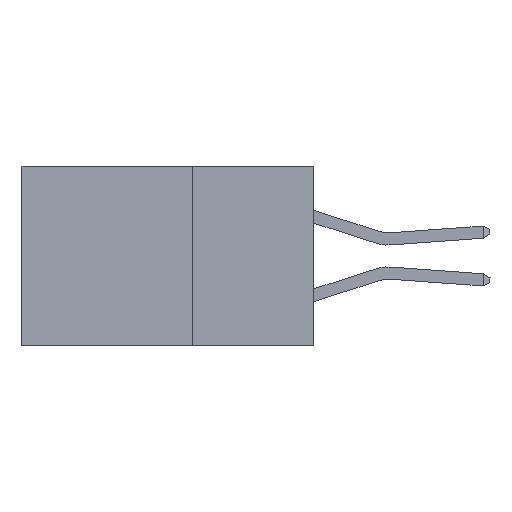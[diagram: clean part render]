
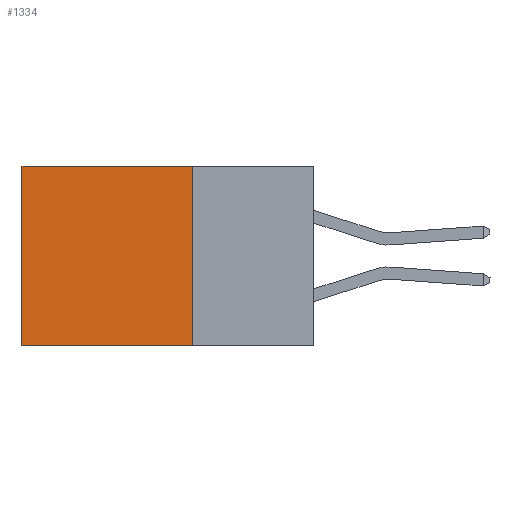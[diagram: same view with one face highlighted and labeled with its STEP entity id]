
A CAD part, left-side view. The second image highlights one B-rep face of the part: STEP entity #1334.
In plain terms, the highlighted planar face has unit normal (-1, 0, 0).
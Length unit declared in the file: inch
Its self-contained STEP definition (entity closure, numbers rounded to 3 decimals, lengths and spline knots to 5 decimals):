
#1334 = ADVANCED_FACE ( 'NONE', ( #14025 ), #2340, .F. ) ;
#2030 = DIRECTION ( 'NONE',  ( 0., 0., -1. ) ) ;
#2246 = DIRECTION ( 'NONE',  ( 1., 0., 0. ) ) ;
#2252 = CARTESIAN_POINT ( 'NONE',  ( 0.2875, 0.25, 0. ) ) ;
#2340 = PLANE ( 'NONE',  #8153 ) ;
#3141 = EDGE_CURVE ( 'NONE', #4321, #3555, #17399, .T. ) ;
#3555 = VERTEX_POINT ( 'NONE', #17788 ) ;
#3614 = CARTESIAN_POINT ( 'NONE',  ( 0.2875, 0.6, 0. ) ) ;
#4321 = VERTEX_POINT ( 'NONE', #3614 ) ;
#4452 = CARTESIAN_POINT ( 'NONE',  ( 0.2875, 0.6, 0. ) ) ;
#6904 = CARTESIAN_POINT ( 'NONE',  ( 0.2875, 0.25, 0. ) ) ;
#7020 = CARTESIAN_POINT ( 'NONE',  ( 0.2875, 0.25, -0.37 ) ) ;
#8153 = AXIS2_PLACEMENT_3D ( 'NONE', #2252, #2246, #2030 ) ;
#8231 = CARTESIAN_POINT ( 'NONE',  ( 0.2875, 0.25, 0. ) ) ;
#9125 = ORIENTED_EDGE ( 'NONE', *, *, #3141, .T. ) ;
#10062 = CARTESIAN_POINT ( 'NONE',  ( 0.2875, 0.25, -0.37 ) ) ;
#10275 = EDGE_CURVE ( 'NONE', #19198, #4321, #13256, .T. ) ;
#10384 = ORIENTED_EDGE ( 'NONE', *, *, #10275, .T. ) ;
#10783 = CARTESIAN_POINT ( 'NONE',  ( 0.2875, 0.25, 0. ) ) ;
#11947 = ORIENTED_EDGE ( 'NONE', *, *, #22106, .F. ) ;
#12358 = VECTOR ( 'NONE', #19217, 39.37008 ) ;
#13256 = LINE ( 'NONE', #6904, #22169 ) ;
#13723 = DIRECTION ( 'NONE',  ( 0., 1., 0. ) ) ;
#14025 = FACE_OUTER_BOUND ( 'NONE', #19454, .T. ) ;
#14488 = VECTOR ( 'NONE', #16910, 39.37008 ) ;
#14865 = ORIENTED_EDGE ( 'NONE', *, *, #15381, .F. ) ;
#15381 = EDGE_CURVE ( 'NONE', #19198, #22263, #19462, .T. ) ;
#15703 = LINE ( 'NONE', #10062, #20112 ) ;
#16910 = DIRECTION ( 'NONE',  ( 0., 0., -1. ) ) ;
#17332 = DIRECTION ( 'NONE',  ( 0., 1., 0. ) ) ;
#17399 = LINE ( 'NONE', #4452, #12358 ) ;
#17788 = CARTESIAN_POINT ( 'NONE',  ( 0.2875, 0.6, -0.37 ) ) ;
#19198 = VERTEX_POINT ( 'NONE', #10783 ) ;
#19217 = DIRECTION ( 'NONE',  ( 0., 0., -1. ) ) ;
#19454 = EDGE_LOOP ( 'NONE', ( #9125, #11947, #14865, #10384 ) ) ;
#19462 = LINE ( 'NONE', #8231, #14488 ) ;
#20112 = VECTOR ( 'NONE', #13723, 39.37008 ) ;
#22106 = EDGE_CURVE ( 'NONE', #22263, #3555, #15703, .T. ) ;
#22169 = VECTOR ( 'NONE', #17332, 39.37008 ) ;
#22263 = VERTEX_POINT ( 'NONE', #7020 ) ;
